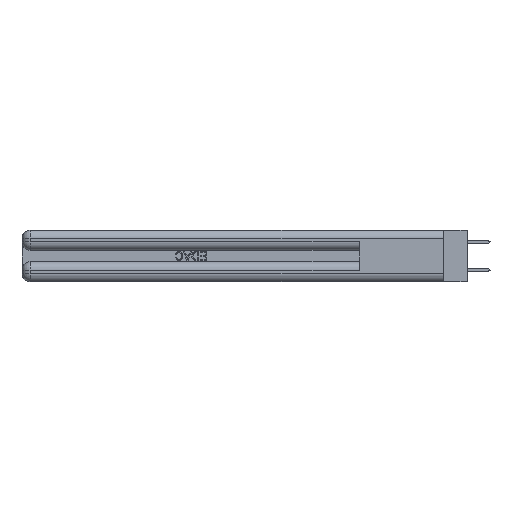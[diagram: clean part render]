
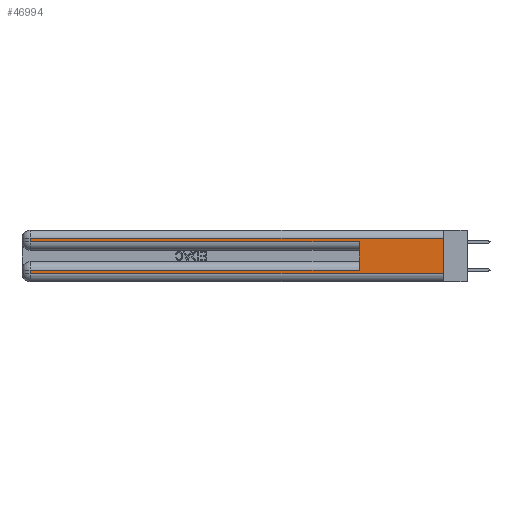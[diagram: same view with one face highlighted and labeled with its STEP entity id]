
A CAD part, left-side view. The second image highlights one B-rep face of the part: STEP entity #46994.
In plain terms, the highlighted planar face has unit normal (-1, 0, 0).
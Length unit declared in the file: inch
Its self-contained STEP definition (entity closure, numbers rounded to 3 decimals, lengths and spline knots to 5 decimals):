
#373 = PLANE ( 'NONE',  #11753 ) ;
#539 = EDGE_CURVE ( 'NONE', #41431, #13832, #29327, .T. ) ;
#791 = DIRECTION ( 'NONE',  ( 0., -1., 0. ) ) ;
#1462 = CARTESIAN_POINT ( 'NONE',  ( 0., 2.94, 0.085 ) ) ;
#2905 = CARTESIAN_POINT ( 'NONE',  ( 0., 0.6, 0.085 ) ) ;
#5649 = LINE ( 'NONE', #10761, #40597 ) ;
#7956 = CARTESIAN_POINT ( 'NONE',  ( 0., 0., 0.37 ) ) ;
#8542 = VERTEX_POINT ( 'NONE', #38712 ) ;
#8850 = LINE ( 'NONE', #33416, #44964 ) ;
#9512 = EDGE_CURVE ( 'NONE', #18323, #8542, #5649, .T. ) ;
#9641 = LINE ( 'NONE', #27951, #17213 ) ;
#10038 = ORIENTED_EDGE ( 'NONE', *, *, #11080, .T. ) ;
#10761 = CARTESIAN_POINT ( 'NONE',  ( 0., 2.94, 0.37 ) ) ;
#11080 = EDGE_CURVE ( 'NONE', #14269, #18323, #15439, .T. ) ;
#11665 = DIRECTION ( 'NONE',  ( 0., 0., -1. ) ) ;
#11753 = AXIS2_PLACEMENT_3D ( 'NONE', #7956, #34063, #11665 ) ;
#13832 = VERTEX_POINT ( 'NONE', #47963 ) ;
#13934 = LINE ( 'NONE', #42587, #43685 ) ;
#14269 = VERTEX_POINT ( 'NONE', #2905 ) ;
#14289 = VECTOR ( 'NONE', #791, 39.37008 ) ;
#15439 = LINE ( 'NONE', #28121, #42831 ) ;
#15629 = EDGE_CURVE ( 'NONE', #45975, #20231, #8850, .T. ) ;
#15864 = CARTESIAN_POINT ( 'NONE',  ( 0., 0., 0.06 ) ) ;
#16408 = CARTESIAN_POINT ( 'NONE',  ( 0., 0., 0.285 ) ) ;
#17213 = VECTOR ( 'NONE', #38946, 39.37008 ) ;
#18323 = VERTEX_POINT ( 'NONE', #1462 ) ;
#20005 = ORIENTED_EDGE ( 'NONE', *, *, #30119, .T. ) ;
#20231 = VERTEX_POINT ( 'NONE', #15864 ) ;
#21104 = ORIENTED_EDGE ( 'NONE', *, *, #15629, .F. ) ;
#22541 = VERTEX_POINT ( 'NONE', #35072 ) ;
#23448 = ORIENTED_EDGE ( 'NONE', *, *, #26441, .F. ) ;
#24388 = DIRECTION ( 'NONE',  ( 0., 1., 0. ) ) ;
#24500 = EDGE_CURVE ( 'NONE', #22541, #41431, #9641, .T. ) ;
#24959 = ORIENTED_EDGE ( 'NONE', *, *, #539, .T. ) ;
#25424 = CARTESIAN_POINT ( 'NONE',  ( 0., 0.6, 0.145 ) ) ;
#25479 = VECTOR ( 'NONE', #32732, 39.37008 ) ;
#26441 = EDGE_CURVE ( 'NONE', #14269, #13832, #35346, .T. ) ;
#27120 = ORIENTED_EDGE ( 'NONE', *, *, #9512, .T. ) ;
#27860 = DIRECTION ( 'NONE',  ( 0., 1., 0. ) ) ;
#27951 = CARTESIAN_POINT ( 'NONE',  ( 0., 2.94, 0.37 ) ) ;
#28121 = CARTESIAN_POINT ( 'NONE',  ( 0., 0., 0.085 ) ) ;
#29327 = LINE ( 'NONE', #16408, #36875 ) ;
#29559 = DIRECTION ( 'NONE',  ( 0., 0., -1. ) ) ;
#30119 = EDGE_CURVE ( 'NONE', #45975, #22541, #13934, .T. ) ;
#32732 = DIRECTION ( 'NONE',  ( 0., 0., 1. ) ) ;
#33416 = CARTESIAN_POINT ( 'NONE',  ( 0., 0., 0.37 ) ) ;
#33577 = DIRECTION ( 'NONE',  ( 0., 0., -1. ) ) ;
#34063 = DIRECTION ( 'NONE',  ( 1., 0., 0. ) ) ;
#34193 = LINE ( 'NONE', #45476, #14289 ) ;
#34360 = CARTESIAN_POINT ( 'NONE',  ( 0., 2.94, 0.285 ) ) ;
#35072 = CARTESIAN_POINT ( 'NONE',  ( 0., 2.94, 0.31 ) ) ;
#35346 = LINE ( 'NONE', #25424, #25479 ) ;
#35902 = CARTESIAN_POINT ( 'NONE',  ( 0., 0., 0.31 ) ) ;
#36514 = ORIENTED_EDGE ( 'NONE', *, *, #40124, .T. ) ;
#36875 = VECTOR ( 'NONE', #38724, 39.37008 ) ;
#38712 = CARTESIAN_POINT ( 'NONE',  ( 0., 2.94, 0.06 ) ) ;
#38724 = DIRECTION ( 'NONE',  ( 0., -1., 0. ) ) ;
#38946 = DIRECTION ( 'NONE',  ( 0., 0., -1. ) ) ;
#39412 = EDGE_LOOP ( 'NONE', ( #21104, #20005, #40326, #24959, #23448, #10038, #27120, #36514 ) ) ;
#40124 = EDGE_CURVE ( 'NONE', #8542, #20231, #34193, .T. ) ;
#40326 = ORIENTED_EDGE ( 'NONE', *, *, #24500, .T. ) ;
#40335 = FACE_OUTER_BOUND ( 'NONE', #39412, .T. ) ;
#40597 = VECTOR ( 'NONE', #29559, 39.37008 ) ;
#41431 = VERTEX_POINT ( 'NONE', #34360 ) ;
#42587 = CARTESIAN_POINT ( 'NONE',  ( 0., 0., 0.31 ) ) ;
#42831 = VECTOR ( 'NONE', #24388, 39.37008 ) ;
#43685 = VECTOR ( 'NONE', #27860, 39.37008 ) ;
#44964 = VECTOR ( 'NONE', #33577, 39.37008 ) ;
#45476 = CARTESIAN_POINT ( 'NONE',  ( 0., 0., 0.06 ) ) ;
#45975 = VERTEX_POINT ( 'NONE', #35902 ) ;
#46994 = ADVANCED_FACE ( 'NONE', ( #40335 ), #373, .F. ) ;
#47963 = CARTESIAN_POINT ( 'NONE',  ( 0., 0.6, 0.285 ) ) ;
